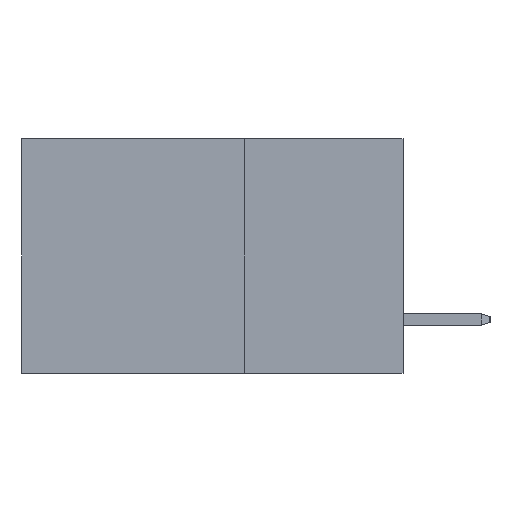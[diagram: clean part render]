
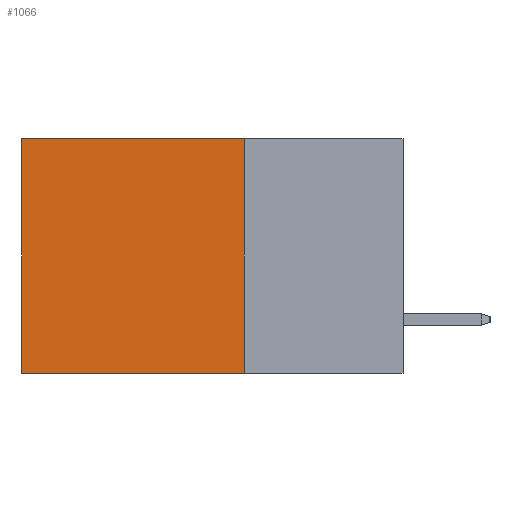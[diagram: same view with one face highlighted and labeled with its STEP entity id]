
A CAD part, left-side view. The second image highlights one B-rep face of the part: STEP entity #1066.
In plain terms, the highlighted planar face has unit normal (-1, 0, 0).
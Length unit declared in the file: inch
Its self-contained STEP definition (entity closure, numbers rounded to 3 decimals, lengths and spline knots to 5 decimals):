
#701 = VECTOR ( 'NONE', #8547, 39.37008 ) ;
#723 = LINE ( 'NONE', #2463, #5636 ) ;
#780 = ORIENTED_EDGE ( 'NONE', *, *, #8157, .F. ) ;
#922 = VERTEX_POINT ( 'NONE', #2112 ) ;
#1066 = ADVANCED_FACE ( 'NONE', ( #5054 ), #9834, .F. ) ;
#1393 = CARTESIAN_POINT ( 'NONE',  ( 0.2875, 0.25, 0. ) ) ;
#1578 = DIRECTION ( 'NONE',  ( 0., 0., -1. ) ) ;
#1727 = ORIENTED_EDGE ( 'NONE', *, *, #3471, .T. ) ;
#2057 = VECTOR ( 'NONE', #6693, 39.37008 ) ;
#2112 = CARTESIAN_POINT ( 'NONE',  ( 0.2875, 0.25, 0. ) ) ;
#2463 = CARTESIAN_POINT ( 'NONE',  ( 0.2875, 0.25, -0.37 ) ) ;
#3142 = VERTEX_POINT ( 'NONE', #4986 ) ;
#3471 = EDGE_CURVE ( 'NONE', #3541, #11844, #5646, .T. ) ;
#3541 = VERTEX_POINT ( 'NONE', #7698 ) ;
#3626 = EDGE_LOOP ( 'NONE', ( #1727, #6175, #780, #4259 ) ) ;
#3653 = LINE ( 'NONE', #5629, #6370 ) ;
#4103 = CARTESIAN_POINT ( 'NONE',  ( 0.2875, 0.6, -0.37 ) ) ;
#4259 = ORIENTED_EDGE ( 'NONE', *, *, #11854, .T. ) ;
#4986 = CARTESIAN_POINT ( 'NONE',  ( 0.2875, 0.25, -0.37 ) ) ;
#5054 = FACE_OUTER_BOUND ( 'NONE', #3626, .T. ) ;
#5629 = CARTESIAN_POINT ( 'NONE',  ( 0.2875, 0.25, 0. ) ) ;
#5636 = VECTOR ( 'NONE', #6995, 39.37008 ) ;
#5646 = LINE ( 'NONE', #9325, #701 ) ;
#6175 = ORIENTED_EDGE ( 'NONE', *, *, #10598, .F. ) ;
#6370 = VECTOR ( 'NONE', #6601, 39.37008 ) ;
#6601 = DIRECTION ( 'NONE',  ( 0., 0., -1. ) ) ;
#6693 = DIRECTION ( 'NONE',  ( 0., 1., 0. ) ) ;
#6751 = LINE ( 'NONE', #7839, #2057 ) ;
#6995 = DIRECTION ( 'NONE',  ( 0., 1., 0. ) ) ;
#7698 = CARTESIAN_POINT ( 'NONE',  ( 0.2875, 0.6, 0. ) ) ;
#7839 = CARTESIAN_POINT ( 'NONE',  ( 0.2875, 0.25, 0. ) ) ;
#8157 = EDGE_CURVE ( 'NONE', #922, #3142, #3653, .T. ) ;
#8547 = DIRECTION ( 'NONE',  ( 0., 0., -1. ) ) ;
#9325 = CARTESIAN_POINT ( 'NONE',  ( 0.2875, 0.6, 0. ) ) ;
#9775 = DIRECTION ( 'NONE',  ( 1., 0., 0. ) ) ;
#9834 = PLANE ( 'NONE',  #9983 ) ;
#9983 = AXIS2_PLACEMENT_3D ( 'NONE', #1393, #9775, #1578 ) ;
#10598 = EDGE_CURVE ( 'NONE', #3142, #11844, #723, .T. ) ;
#11844 = VERTEX_POINT ( 'NONE', #4103 ) ;
#11854 = EDGE_CURVE ( 'NONE', #922, #3541, #6751, .T. ) ;
